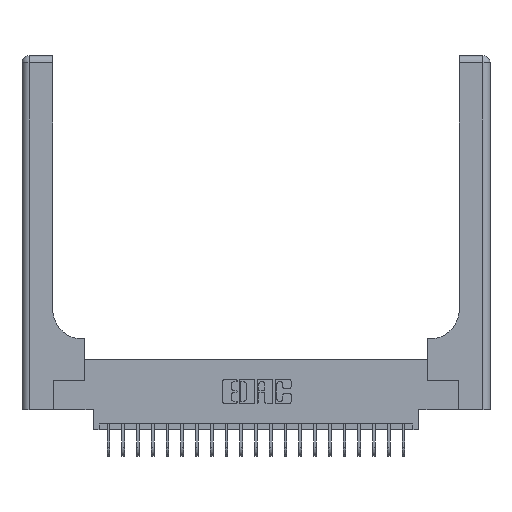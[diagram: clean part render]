
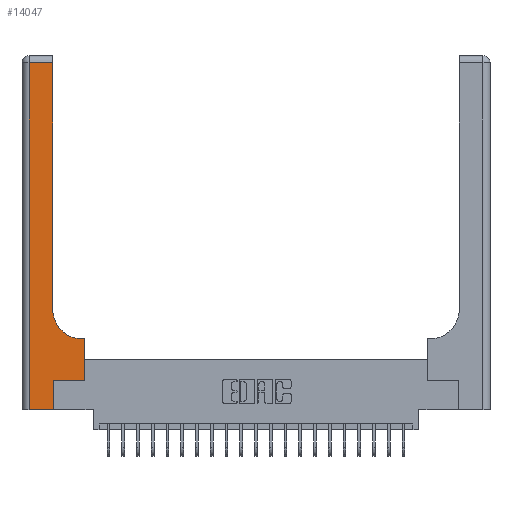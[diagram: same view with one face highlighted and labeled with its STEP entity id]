
A CAD part, top view. The second image highlights one B-rep face of the part: STEP entity #14047.
In plain terms, the highlighted planar face has unit normal (0, 0, 1).
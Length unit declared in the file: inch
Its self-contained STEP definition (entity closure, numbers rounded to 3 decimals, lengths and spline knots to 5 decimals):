
#48 = ORIENTED_EDGE ( 'NONE', *, *, #3369, .T. ) ;
#187 = CARTESIAN_POINT ( 'NONE',  ( 0.528, 0.25, 0.37 ) ) ;
#268 = LINE ( 'NONE', #11474, #6103 ) ;
#449 = CARTESIAN_POINT ( 'NONE',  ( 0.26, 0.85, 0.37 ) ) ;
#1294 = VERTEX_POINT ( 'NONE', #449 ) ;
#1531 = VERTEX_POINT ( 'NONE', #12864 ) ;
#1716 = CARTESIAN_POINT ( 'NONE',  ( 0.26, 0.6, 0.37 ) ) ;
#1771 = LINE ( 'NONE', #5551, #4212 ) ;
#2003 = LINE ( 'NONE', #187, #3323 ) ;
#2257 = LINE ( 'NONE', #7856, #6989 ) ;
#3033 = DIRECTION ( 'NONE',  ( 1., 0., 0. ) ) ;
#3323 = VECTOR ( 'NONE', #20433, 39.37008 ) ;
#3369 = EDGE_CURVE ( 'NONE', #20076, #14662, #3799, .T. ) ;
#3542 = LINE ( 'NONE', #1716, #4386 ) ;
#3784 = DIRECTION ( 'NONE',  ( -1., 0., 0. ) ) ;
#3799 = LINE ( 'NONE', #22350, #6292 ) ;
#4212 = VECTOR ( 'NONE', #9689, 39.37008 ) ;
#4386 = VECTOR ( 'NONE', #3784, 39.37008 ) ;
#4866 = CARTESIAN_POINT ( 'NONE',  ( 0.51, 0.6, 0.37 ) ) ;
#4984 = VERTEX_POINT ( 'NONE', #5643 ) ;
#5551 = CARTESIAN_POINT ( 'NONE',  ( 0., 0., 0.37 ) ) ;
#5643 = CARTESIAN_POINT ( 'NONE',  ( 0.06, 0., 0.37 ) ) ;
#5871 = DIRECTION ( 'NONE',  ( 0., 1., 0. ) ) ;
#5930 = CARTESIAN_POINT ( 'NONE',  ( 0.06, 2.94, 0.37 ) ) ;
#6103 = VECTOR ( 'NONE', #22341, 39.37008 ) ;
#6292 = VECTOR ( 'NONE', #5871, 39.37008 ) ;
#6534 = AXIS2_PLACEMENT_3D ( 'NONE', #13578, #13696, #7942 ) ;
#6782 = EDGE_CURVE ( 'NONE', #16261, #1294, #20443, .T. ) ;
#6821 = ORIENTED_EDGE ( 'NONE', *, *, #14698, .T. ) ;
#6989 = VECTOR ( 'NONE', #20569, 39.37008 ) ;
#7137 = CARTESIAN_POINT ( 'NONE',  ( 0.265, 0.25, 0.37 ) ) ;
#7856 = CARTESIAN_POINT ( 'NONE',  ( 0.265, 0.25, 0.37 ) ) ;
#7942 = DIRECTION ( 'NONE',  ( -1., 0., 0. ) ) ;
#8069 = ORIENTED_EDGE ( 'NONE', *, *, #9399, .T. ) ;
#8169 = ORIENTED_EDGE ( 'NONE', *, *, #10219, .T. ) ;
#8308 = AXIS2_PLACEMENT_3D ( 'NONE', #12311, #10340, #3033 ) ;
#8839 = LINE ( 'NONE', #16300, #18552 ) ;
#9289 = VERTEX_POINT ( 'NONE', #12870 ) ;
#9399 = EDGE_CURVE ( 'NONE', #1531, #21327, #2003, .T. ) ;
#9689 = DIRECTION ( 'NONE',  ( 1., 0., 0. ) ) ;
#10219 = EDGE_CURVE ( 'NONE', #9289, #19536, #22324, .T. ) ;
#10331 = EDGE_LOOP ( 'NONE', ( #14873, #8169, #15803, #6821, #48, #17282, #8069, #11362, #18581 ) ) ;
#10340 = DIRECTION ( 'NONE',  ( 0., 0., -1. ) ) ;
#10656 = EDGE_CURVE ( 'NONE', #1294, #9289, #8839, .T. ) ;
#10675 = CARTESIAN_POINT ( 'NONE',  ( 0.265, 0., 0.37 ) ) ;
#11362 = ORIENTED_EDGE ( 'NONE', *, *, #15665, .T. ) ;
#11474 = CARTESIAN_POINT ( 'NONE',  ( 0.06, 3., 0.37 ) ) ;
#12306 = VECTOR ( 'NONE', #24023, 39.37008 ) ;
#12311 = CARTESIAN_POINT ( 'NONE',  ( 0.51, 0.85, 0.37 ) ) ;
#12864 = CARTESIAN_POINT ( 'NONE',  ( 0.528, 0.25, 0.37 ) ) ;
#12870 = CARTESIAN_POINT ( 'NONE',  ( 0.26, 2.94, 0.37 ) ) ;
#13578 = CARTESIAN_POINT ( 'NONE',  ( 0., 3., 0.37 ) ) ;
#13696 = DIRECTION ( 'NONE',  ( 0., 0., -1. ) ) ;
#14047 = ADVANCED_FACE ( 'NONE', ( #21381 ), #20891, .F. ) ;
#14469 = DIRECTION ( 'NONE',  ( 0., 1., 0. ) ) ;
#14662 = VERTEX_POINT ( 'NONE', #7137 ) ;
#14698 = EDGE_CURVE ( 'NONE', #4984, #20076, #1771, .T. ) ;
#14841 = EDGE_CURVE ( 'NONE', #14662, #1531, #2257, .T. ) ;
#14873 = ORIENTED_EDGE ( 'NONE', *, *, #10656, .T. ) ;
#15255 = CARTESIAN_POINT ( 'NONE',  ( 0.528, 0.6, 0.37 ) ) ;
#15665 = EDGE_CURVE ( 'NONE', #21327, #16261, #3542, .T. ) ;
#15803 = ORIENTED_EDGE ( 'NONE', *, *, #22440, .T. ) ;
#16261 = VERTEX_POINT ( 'NONE', #4866 ) ;
#16300 = CARTESIAN_POINT ( 'NONE',  ( 0.26, 3., 0.37 ) ) ;
#17282 = ORIENTED_EDGE ( 'NONE', *, *, #14841, .T. ) ;
#18552 = VECTOR ( 'NONE', #14469, 39.37008 ) ;
#18581 = ORIENTED_EDGE ( 'NONE', *, *, #6782, .T. ) ;
#19536 = VERTEX_POINT ( 'NONE', #5930 ) ;
#20076 = VERTEX_POINT ( 'NONE', #10675 ) ;
#20258 = CARTESIAN_POINT ( 'NONE',  ( 0., 2.94, 0.37 ) ) ;
#20433 = DIRECTION ( 'NONE',  ( 0., 1., 0. ) ) ;
#20443 = CIRCLE ( 'NONE', #8308, 0.25 ) ;
#20569 = DIRECTION ( 'NONE',  ( 1., 0., 0. ) ) ;
#20891 = PLANE ( 'NONE',  #6534 ) ;
#21327 = VERTEX_POINT ( 'NONE', #15255 ) ;
#21381 = FACE_OUTER_BOUND ( 'NONE', #10331, .T. ) ;
#22324 = LINE ( 'NONE', #20258, #12306 ) ;
#22341 = DIRECTION ( 'NONE',  ( 0., -1., 0. ) ) ;
#22350 = CARTESIAN_POINT ( 'NONE',  ( 0.265, 0., 0.37 ) ) ;
#22440 = EDGE_CURVE ( 'NONE', #19536, #4984, #268, .T. ) ;
#24023 = DIRECTION ( 'NONE',  ( -1., 0., 0. ) ) ;
